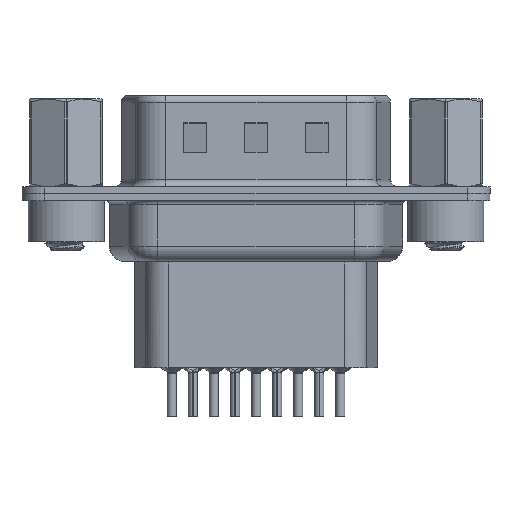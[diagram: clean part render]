
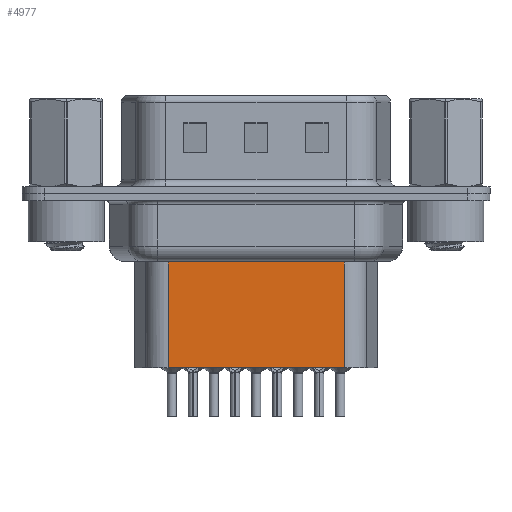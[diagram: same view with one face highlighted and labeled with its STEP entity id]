
A CAD part, front view. The second image highlights one B-rep face of the part: STEP entity #4977.
In plain terms, the highlighted planar face has unit normal (0, -1, 0).
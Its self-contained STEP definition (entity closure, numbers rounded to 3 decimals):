
#1186 = CARTESIAN_POINT ( 'NONE',  ( 6.706, -3.5, -4.097 ) ) ;
#1250 = ORIENTED_EDGE ( 'NONE', *, *, #11881, .T. ) ;
#1285 = CARTESIAN_POINT ( 'NONE',  ( 18.294, -3.5, -4.097 ) ) ;
#2136 = ORIENTED_EDGE ( 'NONE', *, *, #13325, .F. ) ;
#4528 = CARTESIAN_POINT ( 'NONE',  ( 6.459, -3.5, -4.097 ) ) ;
#4977 = ADVANCED_FACE ( 'NONE', ( #12279 ), #14602, .T. ) ;
#5304 = EDGE_CURVE ( 'NONE', #5521, #15393, #13118, .T. ) ;
#5521 = VERTEX_POINT ( 'NONE', #1186 ) ;
#5668 = EDGE_LOOP ( 'NONE', ( #2136, #1250, #11474, #10131 ) ) ;
#8639 = DIRECTION ( 'NONE',  ( 0., 0., -1. ) ) ;
#10131 = ORIENTED_EDGE ( 'NONE', *, *, #12755, .F. ) ;
#10553 = CARTESIAN_POINT ( 'NONE',  ( 6.706, -3.5, -11.45 ) ) ;
#11474 = ORIENTED_EDGE ( 'NONE', *, *, #5304, .T. ) ;
#11711 = DIRECTION ( 'NONE',  ( -1., 0., 0. ) ) ;
#11881 = EDGE_CURVE ( 'NONE', #22776, #5521, #23320, .T. ) ;
#12057 = DIRECTION ( 'NONE',  ( 1., 0., 0. ) ) ;
#12279 = FACE_OUTER_BOUND ( 'NONE', #5668, .T. ) ;
#12604 = DIRECTION ( 'NONE',  ( 0., -1., 0. ) ) ;
#12755 = EDGE_CURVE ( 'NONE', #14623, #15393, #19871, .T. ) ;
#13118 = LINE ( 'NONE', #18234, #21692 ) ;
#13325 = EDGE_CURVE ( 'NONE', #22776, #14623, #16721, .T. ) ;
#13609 = VECTOR ( 'NONE', #11711, 1000. ) ;
#14602 = PLANE ( 'NONE',  #18770 ) ;
#14623 = VERTEX_POINT ( 'NONE', #19470 ) ;
#14993 = VECTOR ( 'NONE', #21461, 1000. ) ;
#15190 = CARTESIAN_POINT ( 'NONE',  ( 6.706, -3.5, -3.1 ) ) ;
#15393 = VERTEX_POINT ( 'NONE', #21601 ) ;
#15697 = CARTESIAN_POINT ( 'NONE',  ( 18.294, -3.5, -3.1 ) ) ;
#16097 = DIRECTION ( 'NONE',  ( 0., 0., -1. ) ) ;
#16721 = LINE ( 'NONE', #15697, #21006 ) ;
#18234 = CARTESIAN_POINT ( 'NONE',  ( 6.706, -3.5, -3.1 ) ) ;
#18770 = AXIS2_PLACEMENT_3D ( 'NONE', #15190, #12604, #12057 ) ;
#19470 = CARTESIAN_POINT ( 'NONE',  ( 18.294, -3.5, -11.45 ) ) ;
#19871 = LINE ( 'NONE', #10553, #14993 ) ;
#21006 = VECTOR ( 'NONE', #8639, 1000. ) ;
#21461 = DIRECTION ( 'NONE',  ( -1., 0., 0. ) ) ;
#21601 = CARTESIAN_POINT ( 'NONE',  ( 6.706, -3.5, -11.45 ) ) ;
#21692 = VECTOR ( 'NONE', #16097, 1000. ) ;
#22776 = VERTEX_POINT ( 'NONE', #1285 ) ;
#23320 = LINE ( 'NONE', #4528, #13609 ) ;
